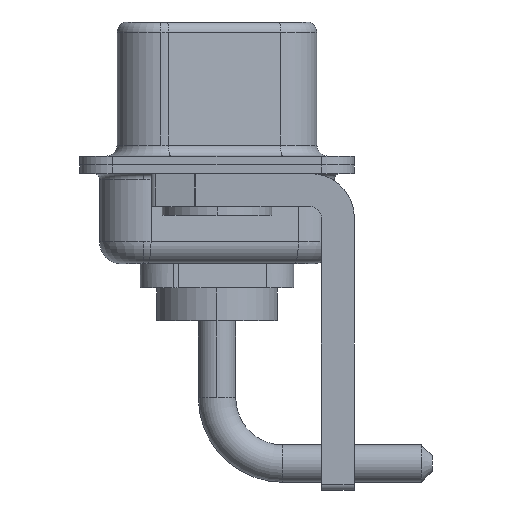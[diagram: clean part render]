
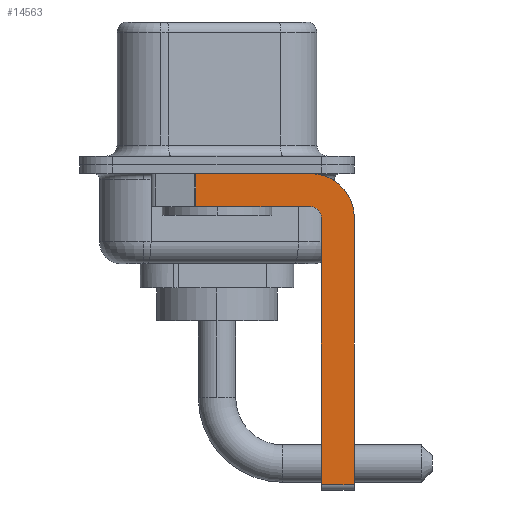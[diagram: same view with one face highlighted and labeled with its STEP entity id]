
A CAD part, left-side view. The second image highlights one B-rep face of the part: STEP entity #14563.
In plain terms, the highlighted planar face has unit normal (-1, 0, 0).
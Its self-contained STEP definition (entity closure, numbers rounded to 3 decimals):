
#707 = EDGE_CURVE ( 'NONE', #5860, #10391, #10742, .T. ) ;
#785 = ORIENTED_EDGE ( 'NONE', *, *, #3808, .F. ) ;
#849 = CARTESIAN_POINT ( 'NONE',  ( -2.9, -6.25, -2.4 ) ) ;
#1208 = CARTESIAN_POINT ( 'NONE',  ( -2.9, -4.75, -14.8 ) ) ;
#1351 = ORIENTED_EDGE ( 'NONE', *, *, #8191, .T. ) ;
#1366 = VERTEX_POINT ( 'NONE', #12374 ) ;
#1372 = VECTOR ( 'NONE', #11583, 1000. ) ;
#1457 = CARTESIAN_POINT ( 'NONE',  ( -2.9, 0.978, -0.4 ) ) ;
#1601 = LINE ( 'NONE', #3858, #1372 ) ;
#1764 = LINE ( 'NONE', #12983, #7303 ) ;
#1880 = VECTOR ( 'NONE', #13575, 1000. ) ;
#2865 = VECTOR ( 'NONE', #4093, 1000. ) ;
#2935 = ORIENTED_EDGE ( 'NONE', *, *, #707, .T. ) ;
#3185 = CARTESIAN_POINT ( 'NONE',  ( -2.9, 0.978, -1.9 ) ) ;
#3581 = DIRECTION ( 'NONE',  ( 0., 0., -1. ) ) ;
#3665 = CARTESIAN_POINT ( 'NONE',  ( -2.9, -4.25, -2.4 ) ) ;
#3737 = CARTESIAN_POINT ( 'NONE',  ( -2.9, -6.25, -2.4 ) ) ;
#3808 = EDGE_CURVE ( 'NONE', #4991, #14258, #14409, .T. ) ;
#3858 = CARTESIAN_POINT ( 'NONE',  ( -2.9, -4.25, -1.9 ) ) ;
#4015 = EDGE_CURVE ( 'NONE', #1366, #10391, #1601, .T. ) ;
#4093 = DIRECTION ( 'NONE',  ( 0., -1., 0. ) ) ;
#4947 = CARTESIAN_POINT ( 'NONE',  ( -2.9, -4.75, -2.4 ) ) ;
#4991 = VERTEX_POINT ( 'NONE', #3737 ) ;
#5100 = VERTEX_POINT ( 'NONE', #10048 ) ;
#5259 = DIRECTION ( 'NONE',  ( 0., 0., -1. ) ) ;
#5752 = CARTESIAN_POINT ( 'NONE',  ( -2.9, -6.25, -14.55 ) ) ;
#5860 = VERTEX_POINT ( 'NONE', #1457 ) ;
#6035 = CARTESIAN_POINT ( 'NONE',  ( -2.9, -4.25, -0.4 ) ) ;
#6268 = EDGE_CURVE ( 'NONE', #11949, #1366, #10447, .T. ) ;
#6291 = DIRECTION ( 'NONE',  ( 0., 0., 1. ) ) ;
#6305 = CIRCLE ( 'NONE', #15079, 2. ) ;
#6422 = CARTESIAN_POINT ( 'NONE',  ( -2.9, 3., -0.4 ) ) ;
#6499 = LINE ( 'NONE', #6422, #2865 ) ;
#6664 = DIRECTION ( 'NONE',  ( 1., 0., 0. ) ) ;
#7303 = VECTOR ( 'NONE', #9417, 1000. ) ;
#8007 = DIRECTION ( 'NONE',  ( 0., 0., -1. ) ) ;
#8191 = EDGE_CURVE ( 'NONE', #5100, #14258, #1764, .T. ) ;
#8489 = ORIENTED_EDGE ( 'NONE', *, *, #4015, .F. ) ;
#8888 = DIRECTION ( 'NONE',  ( 1., 0., 0. ) ) ;
#9347 = ORIENTED_EDGE ( 'NONE', *, *, #10854, .F. ) ;
#9417 = DIRECTION ( 'NONE',  ( 0., -1., 0. ) ) ;
#9644 = AXIS2_PLACEMENT_3D ( 'NONE', #16411, #10240, #13891 ) ;
#10048 = CARTESIAN_POINT ( 'NONE',  ( -2.9, -4.75, -14.55 ) ) ;
#10068 = VERTEX_POINT ( 'NONE', #6035 ) ;
#10240 = DIRECTION ( 'NONE',  ( -1., 0., 0. ) ) ;
#10302 = VECTOR ( 'NONE', #8007, 1000. ) ;
#10391 = VERTEX_POINT ( 'NONE', #13329 ) ;
#10447 = CIRCLE ( 'NONE', #9644, 0.5 ) ;
#10646 = FACE_OUTER_BOUND ( 'NONE', #15252, .T. ) ;
#10742 = LINE ( 'NONE', #3185, #10302 ) ;
#10854 = EDGE_CURVE ( 'NONE', #10068, #4991, #6305, .T. ) ;
#11497 = EDGE_CURVE ( 'NONE', #5100, #11949, #12603, .T. ) ;
#11544 = ORIENTED_EDGE ( 'NONE', *, *, #12493, .F. ) ;
#11583 = DIRECTION ( 'NONE',  ( 0., 1., 0. ) ) ;
#11949 = VERTEX_POINT ( 'NONE', #4947 ) ;
#12374 = CARTESIAN_POINT ( 'NONE',  ( -2.9, -4.25, -1.9 ) ) ;
#12493 = EDGE_CURVE ( 'NONE', #5860, #10068, #6499, .T. ) ;
#12603 = LINE ( 'NONE', #1208, #13216 ) ;
#12983 = CARTESIAN_POINT ( 'NONE',  ( -2.9, -4.25, -14.55 ) ) ;
#13134 = PLANE ( 'NONE',  #15923 ) ;
#13216 = VECTOR ( 'NONE', #6291, 1000. ) ;
#13220 = CARTESIAN_POINT ( 'NONE',  ( -2.9, -4.25, -2.4 ) ) ;
#13329 = CARTESIAN_POINT ( 'NONE',  ( -2.9, 0.978, -1.9 ) ) ;
#13575 = DIRECTION ( 'NONE',  ( 0., 0., -1. ) ) ;
#13891 = DIRECTION ( 'NONE',  ( 0., 0., 1. ) ) ;
#14258 = VERTEX_POINT ( 'NONE', #5752 ) ;
#14409 = LINE ( 'NONE', #849, #1880 ) ;
#14563 = ADVANCED_FACE ( 'NONE', ( #10646 ), #13134, .F. ) ;
#14901 = ORIENTED_EDGE ( 'NONE', *, *, #6268, .F. ) ;
#15079 = AXIS2_PLACEMENT_3D ( 'NONE', #3665, #8888, #3581 ) ;
#15252 = EDGE_LOOP ( 'NONE', ( #11544, #2935, #8489, #14901, #15358, #1351, #785, #9347 ) ) ;
#15358 = ORIENTED_EDGE ( 'NONE', *, *, #11497, .F. ) ;
#15923 = AXIS2_PLACEMENT_3D ( 'NONE', #13220, #6664, #5259 ) ;
#16411 = CARTESIAN_POINT ( 'NONE',  ( -2.9, -4.25, -2.4 ) ) ;
